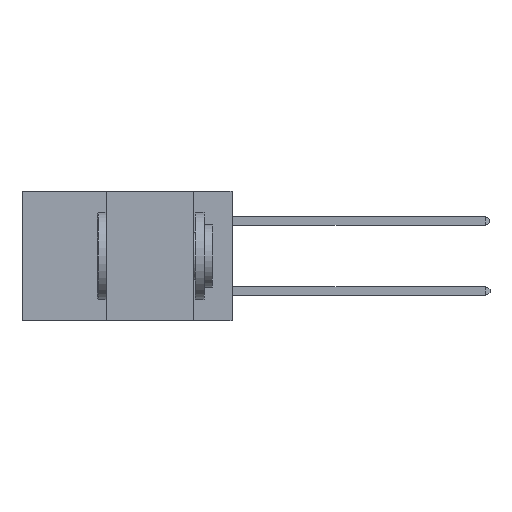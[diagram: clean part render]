
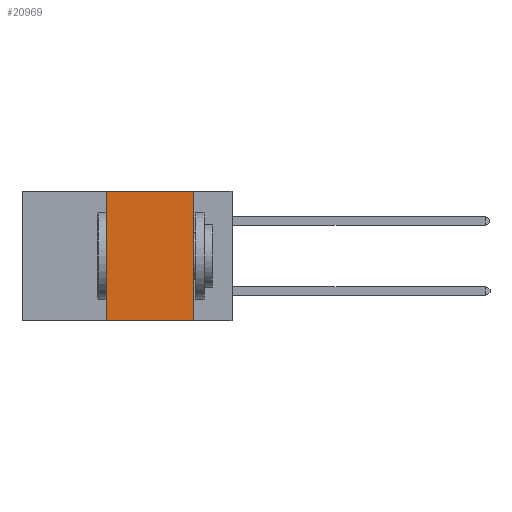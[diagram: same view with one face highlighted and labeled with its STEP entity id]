
A CAD part, left-side view. The second image highlights one B-rep face of the part: STEP entity #20969.
In plain terms, the highlighted planar face has unit normal (-1, 0, 0).
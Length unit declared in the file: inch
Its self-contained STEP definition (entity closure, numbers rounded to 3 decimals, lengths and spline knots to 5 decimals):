
#218 = PLANE ( 'NONE',  #21655 ) ;
#1949 = CARTESIAN_POINT ( 'NONE',  ( 0., 0.6, 0. ) ) ;
#2848 = DIRECTION ( 'NONE',  ( 0., -1., 0. ) ) ;
#3109 = LINE ( 'NONE', #9339, #16939 ) ;
#3240 = LINE ( 'NONE', #13340, #21653 ) ;
#3678 = CARTESIAN_POINT ( 'NONE',  ( 0., 0.11, 0. ) ) ;
#3799 = DIRECTION ( 'NONE',  ( 1., 0., 0. ) ) ;
#3876 = ORIENTED_EDGE ( 'NONE', *, *, #5006, .F. ) ;
#3878 = DIRECTION ( 'NONE',  ( 0., -1., 0. ) ) ;
#5006 = EDGE_CURVE ( 'NONE', #22319, #8117, #10398, .T. ) ;
#5666 = LINE ( 'NONE', #12385, #14396 ) ;
#6641 = EDGE_LOOP ( 'NONE', ( #13185, #3876, #21753, #20680 ) ) ;
#7165 = CARTESIAN_POINT ( 'NONE',  ( 0., 0.36, -0.37 ) ) ;
#8117 = VERTEX_POINT ( 'NONE', #3678 ) ;
#9320 = CARTESIAN_POINT ( 'NONE',  ( 0., 0.36, 0. ) ) ;
#9339 = CARTESIAN_POINT ( 'NONE',  ( 0., 0.11, 0. ) ) ;
#10398 = LINE ( 'NONE', #12671, #14981 ) ;
#10648 = DIRECTION ( 'NONE',  ( 0., 0., 1. ) ) ;
#11698 = EDGE_CURVE ( 'NONE', #20269, #17462, #3240, .T. ) ;
#12121 = FACE_OUTER_BOUND ( 'NONE', #6641, .T. ) ;
#12385 = CARTESIAN_POINT ( 'NONE',  ( 0., 0.36, 0. ) ) ;
#12671 = CARTESIAN_POINT ( 'NONE',  ( 0., 0.6, 0. ) ) ;
#13185 = ORIENTED_EDGE ( 'NONE', *, *, #14399, .F. ) ;
#13340 = CARTESIAN_POINT ( 'NONE',  ( 0., 0.6, -0.37 ) ) ;
#14396 = VECTOR ( 'NONE', #10648, 39.37008 ) ;
#14399 = EDGE_CURVE ( 'NONE', #8117, #17462, #3109, .T. ) ;
#14981 = VECTOR ( 'NONE', #3878, 39.37008 ) ;
#15948 = DIRECTION ( 'NONE',  ( 0., 0., -1. ) ) ;
#16525 = CARTESIAN_POINT ( 'NONE',  ( 0., 0.11, -0.37 ) ) ;
#16939 = VECTOR ( 'NONE', #17749, 39.37008 ) ;
#17462 = VERTEX_POINT ( 'NONE', #16525 ) ;
#17749 = DIRECTION ( 'NONE',  ( 0., 0., -1. ) ) ;
#18573 = EDGE_CURVE ( 'NONE', #20269, #22319, #5666, .T. ) ;
#20269 = VERTEX_POINT ( 'NONE', #7165 ) ;
#20680 = ORIENTED_EDGE ( 'NONE', *, *, #11698, .T. ) ;
#20969 = ADVANCED_FACE ( 'NONE', ( #12121 ), #218, .F. ) ;
#21653 = VECTOR ( 'NONE', #2848, 39.37008 ) ;
#21655 = AXIS2_PLACEMENT_3D ( 'NONE', #1949, #3799, #15948 ) ;
#21753 = ORIENTED_EDGE ( 'NONE', *, *, #18573, .F. ) ;
#22319 = VERTEX_POINT ( 'NONE', #9320 ) ;
